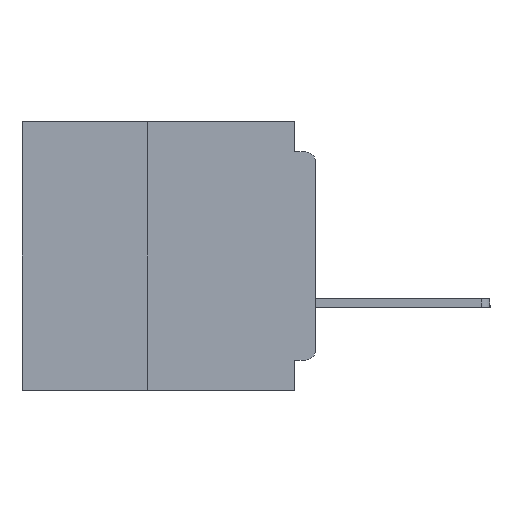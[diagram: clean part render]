
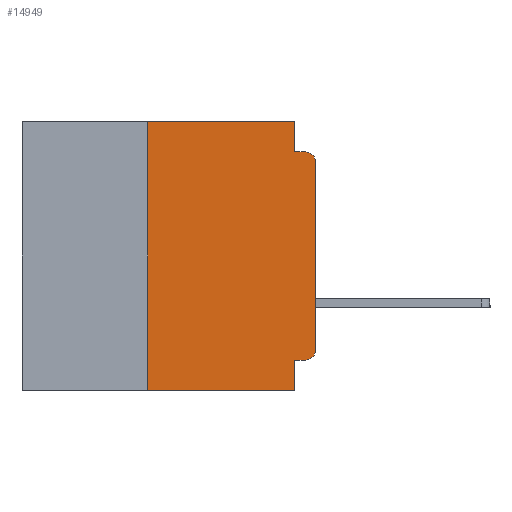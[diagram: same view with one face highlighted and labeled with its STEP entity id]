
A CAD part, left-side view. The second image highlights one B-rep face of the part: STEP entity #14949.
In plain terms, the highlighted planar face has unit normal (-1, 0, 0).
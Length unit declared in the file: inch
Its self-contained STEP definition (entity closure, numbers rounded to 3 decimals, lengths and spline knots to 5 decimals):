
#28 = DIRECTION ( 'NONE',  ( 0., 0., -1. ) ) ;
#121 = CARTESIAN_POINT ( 'NONE',  ( 0., 0.031, 0. ) ) ;
#567 = CARTESIAN_POINT ( 'NONE',  ( 0., 0.031, -0.4 ) ) ;
#1190 = VERTEX_POINT ( 'NONE', #41042 ) ;
#1453 = ORIENTED_EDGE ( 'NONE', *, *, #47945, .F. ) ;
#1962 = VECTOR ( 'NONE', #41694, 39.37008 ) ;
#2066 = EDGE_LOOP ( 'NONE', ( #37194, #2388, #17871, #39370, #29798, #1453, #27575, #14063, #48125, #18796 ) ) ;
#2388 = ORIENTED_EDGE ( 'NONE', *, *, #38314, .T. ) ;
#2501 = VERTEX_POINT ( 'NONE', #121 ) ;
#2571 = DIRECTION ( 'NONE',  ( 0., 0., -1. ) ) ;
#3425 = CARTESIAN_POINT ( 'NONE',  ( 0., 0.015, -0.06 ) ) ;
#4030 = EDGE_CURVE ( 'NONE', #6447, #2501, #40462, .T. ) ;
#4135 = EDGE_CURVE ( 'NONE', #2501, #16177, #4450, .T. ) ;
#4450 = LINE ( 'NONE', #36577, #24602 ) ;
#5738 = DIRECTION ( 'NONE',  ( 0., -1., 0. ) ) ;
#6084 = EDGE_CURVE ( 'NONE', #42555, #37022, #22677, .T. ) ;
#6275 = VERTEX_POINT ( 'NONE', #34361 ) ;
#6447 = VERTEX_POINT ( 'NONE', #39241 ) ;
#7048 = EDGE_CURVE ( 'NONE', #1190, #19173, #17778, .T. ) ;
#7243 = DIRECTION ( 'NONE',  ( 0., 0., -1. ) ) ;
#7969 = VECTOR ( 'NONE', #30766, 39.37008 ) ;
#9041 = DIRECTION ( 'NONE',  ( 0., 1., 0. ) ) ;
#11339 = CARTESIAN_POINT ( 'NONE',  ( 0., 0.437, 0. ) ) ;
#11448 = DIRECTION ( 'NONE',  ( -1., 0., 0. ) ) ;
#11963 = CARTESIAN_POINT ( 'NONE',  ( 0., 0., -0.045 ) ) ;
#12426 = DIRECTION ( 'NONE',  ( 0., -1., 0. ) ) ;
#12897 = CARTESIAN_POINT ( 'NONE',  ( 0., 0., -0.355 ) ) ;
#14063 = ORIENTED_EDGE ( 'NONE', *, *, #32942, .F. ) ;
#14314 = VERTEX_POINT ( 'NONE', #567 ) ;
#14864 = CARTESIAN_POINT ( 'NONE',  ( 0., 0., -0.06 ) ) ;
#14949 = ADVANCED_FACE ( 'NONE', ( #47044 ), #22631, .F. ) ;
#15382 = DIRECTION ( 'NONE',  ( 0., 0., 1. ) ) ;
#15425 = CARTESIAN_POINT ( 'NONE',  ( 0., 0.031, -0.4 ) ) ;
#16177 = VERTEX_POINT ( 'NONE', #41652 ) ;
#17778 = LINE ( 'NONE', #12897, #26607 ) ;
#17871 = ORIENTED_EDGE ( 'NONE', *, *, #32366, .F. ) ;
#18064 = LINE ( 'NONE', #11963, #7969 ) ;
#18796 = ORIENTED_EDGE ( 'NONE', *, *, #28279, .T. ) ;
#19173 = VERTEX_POINT ( 'NONE', #26225 ) ;
#22153 = LINE ( 'NONE', #15425, #1962 ) ;
#22631 = PLANE ( 'NONE',  #35059 ) ;
#22677 = LINE ( 'NONE', #30350, #41410 ) ;
#22785 = DIRECTION ( 'NONE',  ( 1., 0., 0. ) ) ;
#23192 = LINE ( 'NONE', #23680, #41947 ) ;
#23680 = CARTESIAN_POINT ( 'NONE',  ( 0., 0.437, -0.4 ) ) ;
#24602 = VECTOR ( 'NONE', #2571, 39.37008 ) ;
#26225 = CARTESIAN_POINT ( 'NONE',  ( 0., 0.031, -0.355 ) ) ;
#26607 = VECTOR ( 'NONE', #9041, 39.37008 ) ;
#27575 = ORIENTED_EDGE ( 'NONE', *, *, #37961, .T. ) ;
#27702 = VERTEX_POINT ( 'NONE', #34100 ) ;
#28279 = EDGE_CURVE ( 'NONE', #1190, #42555, #38538, .T. ) ;
#28915 = AXIS2_PLACEMENT_3D ( 'NONE', #34039, #11448, #37803 ) ;
#29009 = LINE ( 'NONE', #43871, #47718 ) ;
#29798 = ORIENTED_EDGE ( 'NONE', *, *, #4030, .F. ) ;
#29876 = DIRECTION ( 'NONE',  ( -1., 0., 0. ) ) ;
#30350 = CARTESIAN_POINT ( 'NONE',  ( 0., 0., 0. ) ) ;
#30507 = AXIS2_PLACEMENT_3D ( 'NONE', #3425, #29876, #7243 ) ;
#30766 = DIRECTION ( 'NONE',  ( 0., -1., 0. ) ) ;
#32003 = CARTESIAN_POINT ( 'NONE',  ( 0., 0.437, 0. ) ) ;
#32366 = EDGE_CURVE ( 'NONE', #16177, #27702, #18064, .T. ) ;
#32942 = EDGE_CURVE ( 'NONE', #19173, #14314, #22153, .T. ) ;
#34039 = CARTESIAN_POINT ( 'NONE',  ( 0., 0.015, -0.34 ) ) ;
#34100 = CARTESIAN_POINT ( 'NONE',  ( 0., 0.015, -0.045 ) ) ;
#34290 = CIRCLE ( 'NONE', #30507, 0.015 ) ;
#34361 = CARTESIAN_POINT ( 'NONE',  ( 0., 0.25, -0.4 ) ) ;
#35059 = AXIS2_PLACEMENT_3D ( 'NONE', #11339, #22785, #28 ) ;
#36577 = CARTESIAN_POINT ( 'NONE',  ( 0., 0.031, 0. ) ) ;
#37022 = VERTEX_POINT ( 'NONE', #14864 ) ;
#37194 = ORIENTED_EDGE ( 'NONE', *, *, #6084, .T. ) ;
#37803 = DIRECTION ( 'NONE',  ( 0., 0., -1. ) ) ;
#37961 = EDGE_CURVE ( 'NONE', #6275, #14314, #23192, .T. ) ;
#38122 = VECTOR ( 'NONE', #5738, 39.37008 ) ;
#38314 = EDGE_CURVE ( 'NONE', #37022, #27702, #34290, .T. ) ;
#38538 = CIRCLE ( 'NONE', #28915, 0.015 ) ;
#39241 = CARTESIAN_POINT ( 'NONE',  ( 0., 0.25, 0. ) ) ;
#39370 = ORIENTED_EDGE ( 'NONE', *, *, #4135, .F. ) ;
#39814 = CARTESIAN_POINT ( 'NONE',  ( 0., 0., -0.34 ) ) ;
#40462 = LINE ( 'NONE', #32003, #38122 ) ;
#41042 = CARTESIAN_POINT ( 'NONE',  ( 0., 0.015, -0.355 ) ) ;
#41410 = VECTOR ( 'NONE', #15382, 39.37008 ) ;
#41652 = CARTESIAN_POINT ( 'NONE',  ( 0., 0.031, -0.045 ) ) ;
#41694 = DIRECTION ( 'NONE',  ( 0., 0., -1. ) ) ;
#41947 = VECTOR ( 'NONE', #12426, 39.37008 ) ;
#42555 = VERTEX_POINT ( 'NONE', #39814 ) ;
#43871 = CARTESIAN_POINT ( 'NONE',  ( 0., 0.25, -0.4 ) ) ;
#47044 = FACE_OUTER_BOUND ( 'NONE', #2066, .T. ) ;
#47615 = DIRECTION ( 'NONE',  ( 0., 0., 1. ) ) ;
#47718 = VECTOR ( 'NONE', #47615, 39.37008 ) ;
#47945 = EDGE_CURVE ( 'NONE', #6275, #6447, #29009, .T. ) ;
#48125 = ORIENTED_EDGE ( 'NONE', *, *, #7048, .F. ) ;
